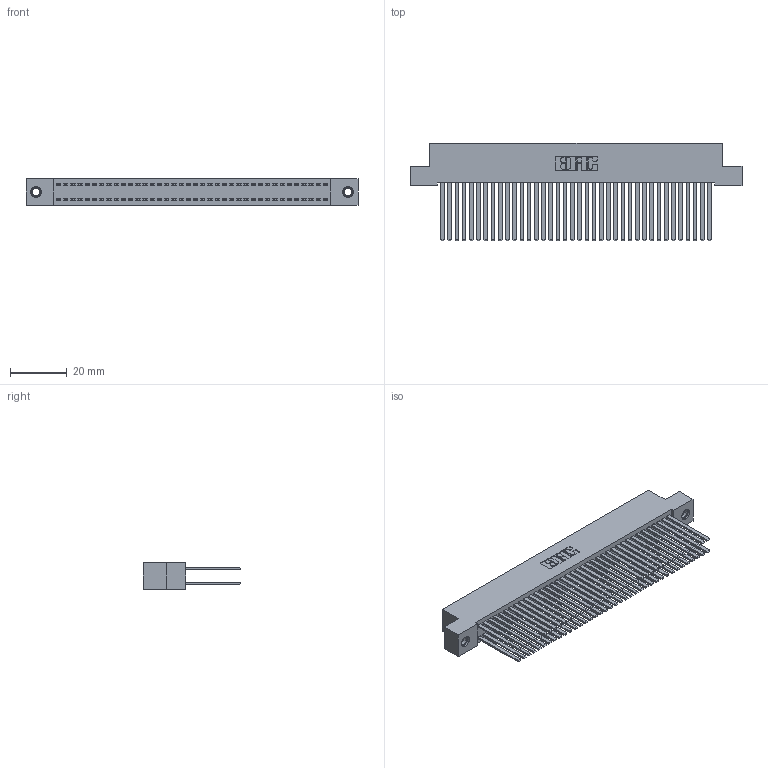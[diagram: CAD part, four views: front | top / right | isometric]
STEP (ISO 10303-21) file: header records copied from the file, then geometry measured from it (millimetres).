
FILE_DESCRIPTION (( 'STEP AP203' ), '1' );
FILE_NAME ('392-076-544-207.STEP', '2019-10-09T13:35:51', ( '' ), ( '' ), 'SwSTEP 2.0', 'SolidWorks 2016', '' );
FILE_SCHEMA (( 'CONFIG_CONTROL_DESIGN' ));
Length unit declared in the file: inch
Products named in the file (4): 345-292-001_345-293-144; 345-250-001_345-250-005-103; 392-076-544-207; 342 Part_TI
Assembly tree (79 placements, depth 2):
  392-076-544-207
    342 Part_TI
    345-292-001_345-293-144  x76
    345-250-001_345-250-005-103  x2
Bounding box: 116.84 x 34.3 x 9.4 mm (x, y, z)
Volume: 11531.8 mm3; surface area: 21648.5 mm2
Topology: 79 solids, 79 shells, 3666 faces, 10847 edges, 7122 vertices
Faces by surface type: plane 2530, cylinder 1120, cone 12, torus 4
Entity records: 25834 total; most frequent: CARTESIAN_POINT 4265, ORIENTED_EDGE 4194, DIRECTION 3679, EDGE_CURVE 2097, LINE 1953, VECTOR 1953, VERTEX_POINT 1392, AXIS2_PLACEMENT_3D 863
